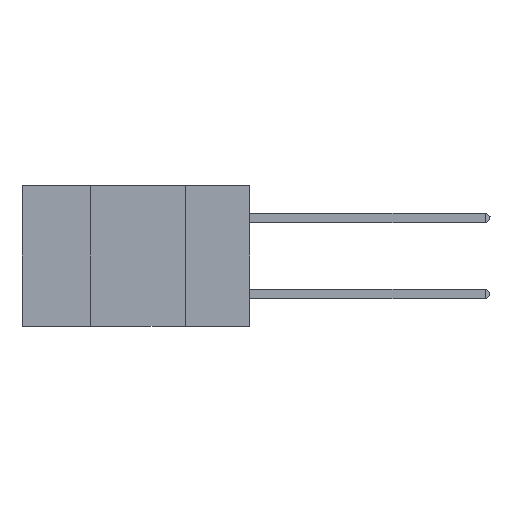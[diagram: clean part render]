
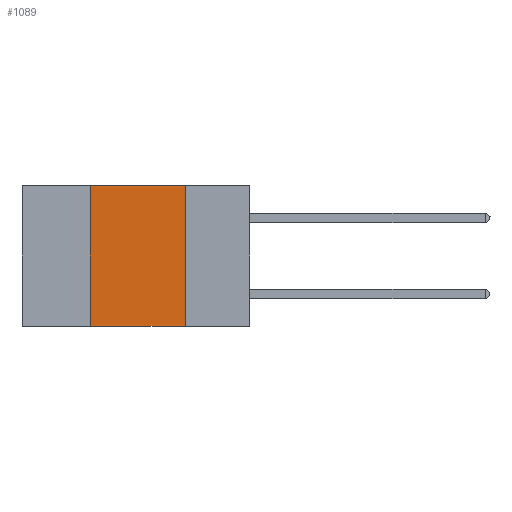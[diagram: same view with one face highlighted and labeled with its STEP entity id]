
A CAD part, left-side view. The second image highlights one B-rep face of the part: STEP entity #1089.
In plain terms, the highlighted planar face has unit normal (-1, 0, 0).
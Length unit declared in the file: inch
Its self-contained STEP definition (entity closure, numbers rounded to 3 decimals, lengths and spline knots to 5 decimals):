
#534 = VERTEX_POINT ( 'NONE', #2755 ) ;
#832 = VECTOR ( 'NONE', #5518, 39.37008 ) ;
#1089 = ADVANCED_FACE ( 'NONE', ( #7039 ), #8131, .F. ) ;
#2395 = CARTESIAN_POINT ( 'NONE',  ( 0., 0.17, 0. ) ) ;
#2399 = CARTESIAN_POINT ( 'NONE',  ( 0., 0.42, 0. ) ) ;
#2504 = ORIENTED_EDGE ( 'NONE', *, *, #10146, .T. ) ;
#2755 = CARTESIAN_POINT ( 'NONE',  ( 0., 0.17, -0.37 ) ) ;
#2911 = DIRECTION ( 'NONE',  ( 0., 0., 1. ) ) ;
#3222 = ORIENTED_EDGE ( 'NONE', *, *, #3561, .F. ) ;
#3561 = EDGE_CURVE ( 'NONE', #9740, #534, #4593, .T. ) ;
#3690 = EDGE_CURVE ( 'NONE', #5636, #9740, #9812, .T. ) ;
#3830 = VERTEX_POINT ( 'NONE', #6554 ) ;
#3867 = LINE ( 'NONE', #7113, #7599 ) ;
#3949 = DIRECTION ( 'NONE',  ( 0., 0., -1. ) ) ;
#4364 = VECTOR ( 'NONE', #9974, 39.37008 ) ;
#4445 = ORIENTED_EDGE ( 'NONE', *, *, #7542, .F. ) ;
#4593 = LINE ( 'NONE', #2395, #4364 ) ;
#4689 = CARTESIAN_POINT ( 'NONE',  ( 0., 0.6, 0. ) ) ;
#5518 = DIRECTION ( 'NONE',  ( 0., -1., 0. ) ) ;
#5636 = VERTEX_POINT ( 'NONE', #2399 ) ;
#5903 = CARTESIAN_POINT ( 'NONE',  ( 0., 0.17, 0. ) ) ;
#6402 = CARTESIAN_POINT ( 'NONE',  ( 0., 0.6, -0.37 ) ) ;
#6554 = CARTESIAN_POINT ( 'NONE',  ( 0., 0.42, -0.37 ) ) ;
#7039 = FACE_OUTER_BOUND ( 'NONE', #10584, .T. ) ;
#7113 = CARTESIAN_POINT ( 'NONE',  ( 0., 0.42, 0. ) ) ;
#7320 = CARTESIAN_POINT ( 'NONE',  ( 0., 0.6, 0. ) ) ;
#7490 = AXIS2_PLACEMENT_3D ( 'NONE', #7320, #9025, #3949 ) ;
#7542 = EDGE_CURVE ( 'NONE', #3830, #5636, #3867, .T. ) ;
#7599 = VECTOR ( 'NONE', #2911, 39.37008 ) ;
#8131 = PLANE ( 'NONE',  #7490 ) ;
#9025 = DIRECTION ( 'NONE',  ( 1., 0., 0. ) ) ;
#9665 = ORIENTED_EDGE ( 'NONE', *, *, #3690, .F. ) ;
#9740 = VERTEX_POINT ( 'NONE', #5903 ) ;
#9812 = LINE ( 'NONE', #4689, #10730 ) ;
#9974 = DIRECTION ( 'NONE',  ( 0., 0., -1. ) ) ;
#10047 = LINE ( 'NONE', #6402, #832 ) ;
#10146 = EDGE_CURVE ( 'NONE', #3830, #534, #10047, .T. ) ;
#10584 = EDGE_LOOP ( 'NONE', ( #3222, #9665, #4445, #2504 ) ) ;
#10686 = DIRECTION ( 'NONE',  ( 0., -1., 0. ) ) ;
#10730 = VECTOR ( 'NONE', #10686, 39.37008 ) ;
